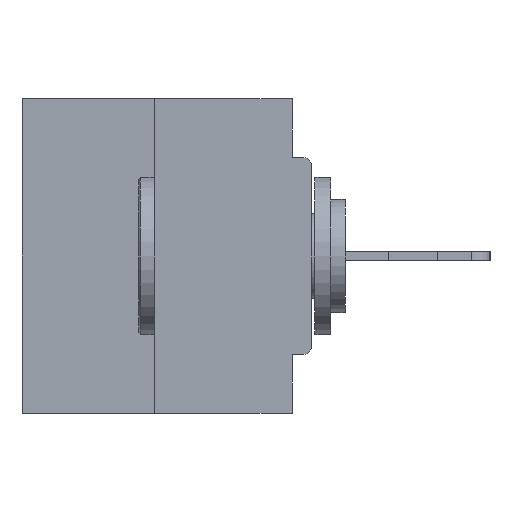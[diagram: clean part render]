
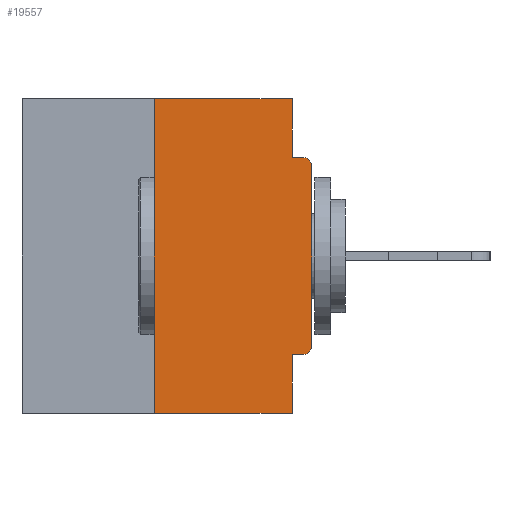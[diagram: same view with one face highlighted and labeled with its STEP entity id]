
A CAD part, left-side view. The second image highlights one B-rep face of the part: STEP entity #19557.
In plain terms, the highlighted planar face has unit normal (-1, 0, 0).
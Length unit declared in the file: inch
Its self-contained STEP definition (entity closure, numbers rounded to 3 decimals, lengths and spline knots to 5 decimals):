
#1502 = DIRECTION ( 'NONE',  ( 0., 0., -1. ) ) ;
#2043 = CARTESIAN_POINT ( 'NONE',  ( 0., 0., 0. ) ) ;
#2471 = EDGE_CURVE ( 'NONE', #25352, #4113, #26597, .T. ) ;
#2735 = FACE_OUTER_BOUND ( 'NONE', #4592, .T. ) ;
#2741 = CARTESIAN_POINT ( 'NONE',  ( 0., 0.015, -0.3915 ) ) ;
#4094 = EDGE_CURVE ( 'NONE', #25352, #29943, #14011, .T. ) ;
#4113 = VERTEX_POINT ( 'NONE', #21461 ) ;
#4476 = LINE ( 'NONE', #13248, #16054 ) ;
#4523 = VERTEX_POINT ( 'NONE', #11255 ) ;
#4592 = EDGE_LOOP ( 'NONE', ( #27936, #23307, #29781, #30343, #25005, #8228, #7022, #23601, #24809, #13476 ) ) ;
#5231 = DIRECTION ( 'NONE',  ( 0., 0., -1. ) ) ;
#5304 = VERTEX_POINT ( 'NONE', #19127 ) ;
#5833 = VERTEX_POINT ( 'NONE', #29487 ) ;
#5858 = AXIS2_PLACEMENT_3D ( 'NONE', #30636, #16319, #1502 ) ;
#6839 = CARTESIAN_POINT ( 'NONE',  ( 0., 0.031, -0.0935 ) ) ;
#7022 = ORIENTED_EDGE ( 'NONE', *, *, #24132, .T. ) ;
#8228 = ORIENTED_EDGE ( 'NONE', *, *, #25492, .T. ) ;
#8551 = VECTOR ( 'NONE', #14862, 39.37008 ) ;
#8739 = VERTEX_POINT ( 'NONE', #14730 ) ;
#8967 = CARTESIAN_POINT ( 'NONE',  ( 0., 0.25, 0. ) ) ;
#9724 = LINE ( 'NONE', #28556, #17044 ) ;
#10067 = EDGE_CURVE ( 'NONE', #19043, #4523, #15890, .T. ) ;
#11255 = CARTESIAN_POINT ( 'NONE',  ( 0., 0.015, -0.0935 ) ) ;
#12163 = CARTESIAN_POINT ( 'NONE',  ( 0., 0., -0.4065 ) ) ;
#12402 = CARTESIAN_POINT ( 'NONE',  ( 0., 0., -0.0935 ) ) ;
#12968 = CARTESIAN_POINT ( 'NONE',  ( 0., 0.031, 0. ) ) ;
#13248 = CARTESIAN_POINT ( 'NONE',  ( 0., 0.031, 0. ) ) ;
#13476 = ORIENTED_EDGE ( 'NONE', *, *, #17043, .F. ) ;
#13632 = CARTESIAN_POINT ( 'NONE',  ( 0., 0.015, -0.1085 ) ) ;
#14010 = VERTEX_POINT ( 'NONE', #24348 ) ;
#14011 = LINE ( 'NONE', #24804, #21258 ) ;
#14730 = CARTESIAN_POINT ( 'NONE',  ( 0., 0.015, -0.4065 ) ) ;
#14862 = DIRECTION ( 'NONE',  ( 0., -1., 0. ) ) ;
#15890 = LINE ( 'NONE', #12402, #8551 ) ;
#16054 = VECTOR ( 'NONE', #20614, 39.37008 ) ;
#16106 = DIRECTION ( 'NONE',  ( 0., 0., -1. ) ) ;
#16319 = DIRECTION ( 'NONE',  ( 1., 0., 0. ) ) ;
#16599 = LINE ( 'NONE', #12163, #18134 ) ;
#17043 = EDGE_CURVE ( 'NONE', #26666, #19043, #4476, .T. ) ;
#17044 = VECTOR ( 'NONE', #30908, 39.37008 ) ;
#17915 = AXIS2_PLACEMENT_3D ( 'NONE', #13632, #30443, #16106 ) ;
#18134 = VECTOR ( 'NONE', #31375, 39.37008 ) ;
#19043 = VERTEX_POINT ( 'NONE', #6839 ) ;
#19127 = CARTESIAN_POINT ( 'NONE',  ( 0., 0., -0.1085 ) ) ;
#19557 = ADVANCED_FACE ( 'NONE', ( #2735 ), #28295, .F. ) ;
#19959 = DIRECTION ( 'NONE',  ( -1., 0., 0. ) ) ;
#20115 = LINE ( 'NONE', #2043, #25721 ) ;
#20229 = VECTOR ( 'NONE', #28851, 39.37008 ) ;
#20614 = DIRECTION ( 'NONE',  ( 0., 0., -1. ) ) ;
#20735 = CARTESIAN_POINT ( 'NONE',  ( 0., 0.031, -0.5 ) ) ;
#20802 = DIRECTION ( 'NONE',  ( 0., 0., 1. ) ) ;
#21258 = VECTOR ( 'NONE', #20802, 39.37008 ) ;
#21461 = CARTESIAN_POINT ( 'NONE',  ( 0., 0.031, -0.5 ) ) ;
#21720 = DIRECTION ( 'NONE',  ( 0., 0., 1. ) ) ;
#21747 = AXIS2_PLACEMENT_3D ( 'NONE', #2741, #19959, #5231 ) ;
#23153 = DIRECTION ( 'NONE',  ( 0., 0., -1. ) ) ;
#23307 = ORIENTED_EDGE ( 'NONE', *, *, #4094, .F. ) ;
#23601 = ORIENTED_EDGE ( 'NONE', *, *, #25782, .T. ) ;
#24132 = EDGE_CURVE ( 'NONE', #5833, #5304, #20115, .T. ) ;
#24348 = CARTESIAN_POINT ( 'NONE',  ( 0., 0.031, -0.4065 ) ) ;
#24713 = EDGE_CURVE ( 'NONE', #29943, #26666, #9724, .T. ) ;
#24804 = CARTESIAN_POINT ( 'NONE',  ( 0., 0.25, 0. ) ) ;
#24809 = ORIENTED_EDGE ( 'NONE', *, *, #10067, .F. ) ;
#25005 = ORIENTED_EDGE ( 'NONE', *, *, #25375, .F. ) ;
#25297 = CIRCLE ( 'NONE', #21747, 0.015 ) ;
#25352 = VERTEX_POINT ( 'NONE', #28832 ) ;
#25375 = EDGE_CURVE ( 'NONE', #8739, #14010, #16599, .T. ) ;
#25492 = EDGE_CURVE ( 'NONE', #8739, #5833, #25297, .T. ) ;
#25721 = VECTOR ( 'NONE', #21720, 39.37008 ) ;
#25782 = EDGE_CURVE ( 'NONE', #5304, #4523, #30465, .T. ) ;
#26597 = LINE ( 'NONE', #28287, #20229 ) ;
#26666 = VERTEX_POINT ( 'NONE', #12968 ) ;
#27936 = ORIENTED_EDGE ( 'NONE', *, *, #24713, .F. ) ;
#28101 = LINE ( 'NONE', #20735, #29587 ) ;
#28287 = CARTESIAN_POINT ( 'NONE',  ( 0., 0.46, -0.5 ) ) ;
#28295 = PLANE ( 'NONE',  #5858 ) ;
#28556 = CARTESIAN_POINT ( 'NONE',  ( 0., 0.46, 0. ) ) ;
#28832 = CARTESIAN_POINT ( 'NONE',  ( 0., 0.25, -0.5 ) ) ;
#28851 = DIRECTION ( 'NONE',  ( 0., -1., 0. ) ) ;
#29487 = CARTESIAN_POINT ( 'NONE',  ( 0., 0., -0.3915 ) ) ;
#29587 = VECTOR ( 'NONE', #23153, 39.37008 ) ;
#29781 = ORIENTED_EDGE ( 'NONE', *, *, #2471, .T. ) ;
#29824 = EDGE_CURVE ( 'NONE', #14010, #4113, #28101, .T. ) ;
#29943 = VERTEX_POINT ( 'NONE', #8967 ) ;
#30343 = ORIENTED_EDGE ( 'NONE', *, *, #29824, .F. ) ;
#30443 = DIRECTION ( 'NONE',  ( -1., 0., 0. ) ) ;
#30465 = CIRCLE ( 'NONE', #17915, 0.015 ) ;
#30636 = CARTESIAN_POINT ( 'NONE',  ( 0., 0.46, 0. ) ) ;
#30908 = DIRECTION ( 'NONE',  ( 0., -1., 0. ) ) ;
#31375 = DIRECTION ( 'NONE',  ( 0., 1., 0. ) ) ;
